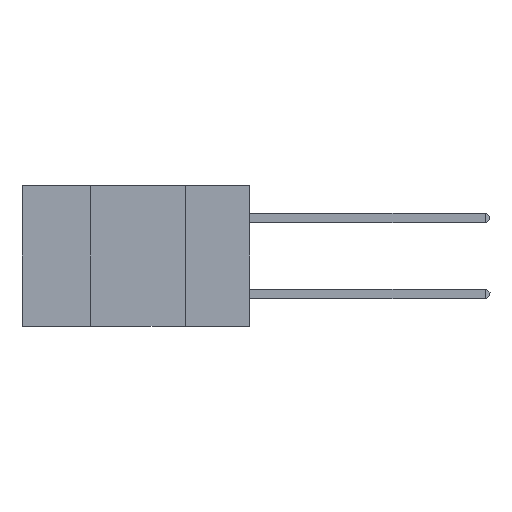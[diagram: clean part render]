
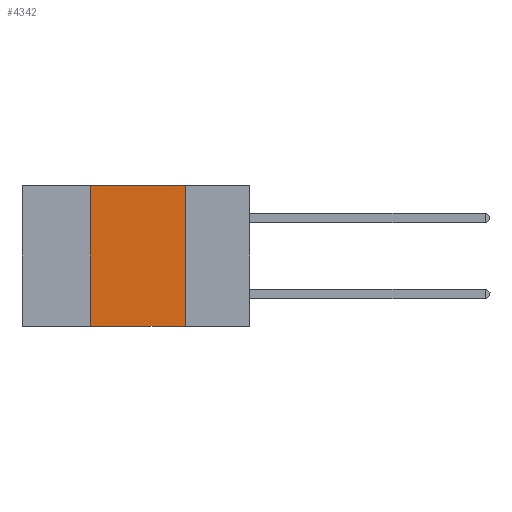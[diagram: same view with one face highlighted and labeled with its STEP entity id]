
A CAD part, left-side view. The second image highlights one B-rep face of the part: STEP entity #4342.
In plain terms, the highlighted planar face has unit normal (-1, 0, 0).
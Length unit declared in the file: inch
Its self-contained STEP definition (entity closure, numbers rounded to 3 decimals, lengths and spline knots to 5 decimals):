
#773 = EDGE_CURVE ( 'NONE', #3305, #5014, #4187, .T. ) ;
#1047 = DIRECTION ( 'NONE',  ( 0., 0., 1. ) ) ;
#1185 = CARTESIAN_POINT ( 'NONE',  ( 0., 0.42, 0. ) ) ;
#1471 = DIRECTION ( 'NONE',  ( 0., 0., -1. ) ) ;
#1873 = CARTESIAN_POINT ( 'NONE',  ( 0., 0.42, 0. ) ) ;
#2050 = VECTOR ( 'NONE', #7960, 39.37008 ) ;
#2200 = CARTESIAN_POINT ( 'NONE',  ( 0., 0.6, -0.37 ) ) ;
#2221 = DIRECTION ( 'NONE',  ( 1., 0., 0. ) ) ;
#2287 = EDGE_CURVE ( 'NONE', #7731, #5014, #3851, .T. ) ;
#2489 = EDGE_CURVE ( 'NONE', #4814, #3305, #3455, .T. ) ;
#2947 = EDGE_LOOP ( 'NONE', ( #6158, #7098, #3974, #8048 ) ) ;
#3305 = VERTEX_POINT ( 'NONE', #4855 ) ;
#3455 = LINE ( 'NONE', #7323, #6337 ) ;
#3732 = VECTOR ( 'NONE', #3792, 39.37008 ) ;
#3792 = DIRECTION ( 'NONE',  ( 0., -1., 0. ) ) ;
#3851 = LINE ( 'NONE', #2200, #3732 ) ;
#3974 = ORIENTED_EDGE ( 'NONE', *, *, #4536, .F. ) ;
#4187 = LINE ( 'NONE', #7354, #2050 ) ;
#4342 = ADVANCED_FACE ( 'NONE', ( #8524 ), #10164, .F. ) ;
#4536 = EDGE_CURVE ( 'NONE', #7731, #4814, #9624, .T. ) ;
#4649 = CARTESIAN_POINT ( 'NONE',  ( 0., 0.17, -0.37 ) ) ;
#4814 = VERTEX_POINT ( 'NONE', #1185 ) ;
#4855 = CARTESIAN_POINT ( 'NONE',  ( 0., 0.17, 0. ) ) ;
#5014 = VERTEX_POINT ( 'NONE', #4649 ) ;
#6158 = ORIENTED_EDGE ( 'NONE', *, *, #773, .F. ) ;
#6337 = VECTOR ( 'NONE', #8941, 39.37008 ) ;
#7098 = ORIENTED_EDGE ( 'NONE', *, *, #2489, .F. ) ;
#7323 = CARTESIAN_POINT ( 'NONE',  ( 0., 0.6, 0. ) ) ;
#7354 = CARTESIAN_POINT ( 'NONE',  ( 0., 0.17, 0. ) ) ;
#7554 = AXIS2_PLACEMENT_3D ( 'NONE', #9381, #2221, #1471 ) ;
#7591 = CARTESIAN_POINT ( 'NONE',  ( 0., 0.42, -0.37 ) ) ;
#7731 = VERTEX_POINT ( 'NONE', #7591 ) ;
#7917 = VECTOR ( 'NONE', #1047, 39.37008 ) ;
#7960 = DIRECTION ( 'NONE',  ( 0., 0., -1. ) ) ;
#8048 = ORIENTED_EDGE ( 'NONE', *, *, #2287, .T. ) ;
#8524 = FACE_OUTER_BOUND ( 'NONE', #2947, .T. ) ;
#8941 = DIRECTION ( 'NONE',  ( 0., -1., 0. ) ) ;
#9381 = CARTESIAN_POINT ( 'NONE',  ( 0., 0.6, 0. ) ) ;
#9624 = LINE ( 'NONE', #1873, #7917 ) ;
#10164 = PLANE ( 'NONE',  #7554 ) ;
